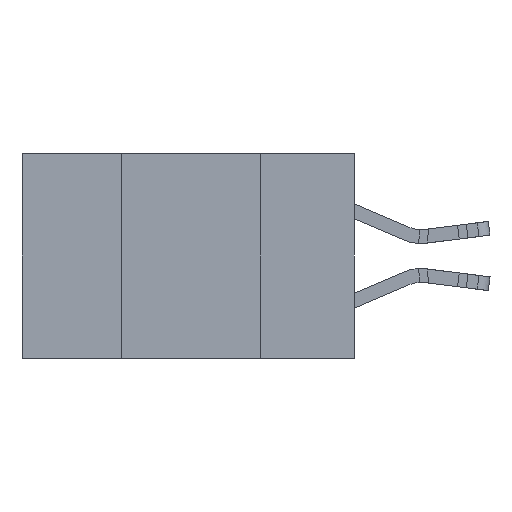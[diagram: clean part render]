
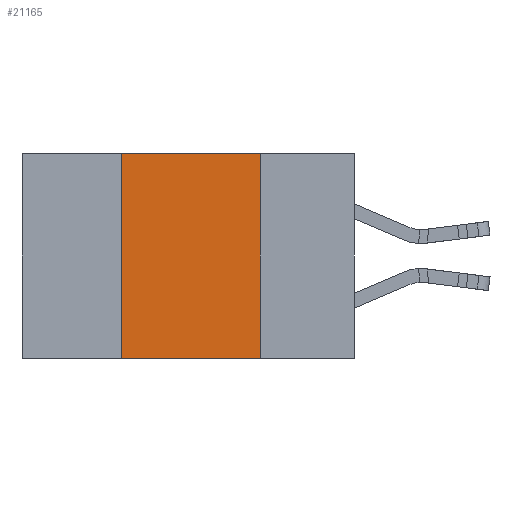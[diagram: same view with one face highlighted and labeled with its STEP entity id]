
A CAD part, left-side view. The second image highlights one B-rep face of the part: STEP entity #21165.
In plain terms, the highlighted planar face has unit normal (-1, 0, 0).
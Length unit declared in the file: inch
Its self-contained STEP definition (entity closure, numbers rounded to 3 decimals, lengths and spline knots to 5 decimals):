
#980 = ORIENTED_EDGE ( 'NONE', *, *, #19626, .T. ) ;
#2289 = ORIENTED_EDGE ( 'NONE', *, *, #3770, .F. ) ;
#3202 = VECTOR ( 'NONE', #24590, 39.37008 ) ;
#3365 = AXIS2_PLACEMENT_3D ( 'NONE', #32123, #9654, #14786 ) ;
#3557 = ORIENTED_EDGE ( 'NONE', *, *, #28721, .F. ) ;
#3770 = EDGE_CURVE ( 'NONE', #24191, #9089, #25655, .T. ) ;
#5657 = CARTESIAN_POINT ( 'NONE',  ( 0., 0.6, 0. ) ) ;
#6574 = CARTESIAN_POINT ( 'NONE',  ( 0., 0.42, -0.37 ) ) ;
#7060 = CARTESIAN_POINT ( 'NONE',  ( 0., 0.42, 0. ) ) ;
#9089 = VERTEX_POINT ( 'NONE', #14503 ) ;
#9654 = DIRECTION ( 'NONE',  ( 1., 0., 0. ) ) ;
#10833 = CARTESIAN_POINT ( 'NONE',  ( 0., 0.17, -0.37 ) ) ;
#10866 = CARTESIAN_POINT ( 'NONE',  ( 0., 0.42, 0. ) ) ;
#11649 = DIRECTION ( 'NONE',  ( 0., -1., 0. ) ) ;
#11809 = EDGE_LOOP ( 'NONE', ( #31295, #2289, #3557, #980 ) ) ;
#12265 = PLANE ( 'NONE',  #3365 ) ;
#14009 = FACE_OUTER_BOUND ( 'NONE', #11809, .T. ) ;
#14503 = CARTESIAN_POINT ( 'NONE',  ( 0., 0.17, 0. ) ) ;
#14786 = DIRECTION ( 'NONE',  ( 0., 0., -1. ) ) ;
#14924 = LINE ( 'NONE', #7060, #3202 ) ;
#15741 = DIRECTION ( 'NONE',  ( 0., -1., 0. ) ) ;
#16377 = CARTESIAN_POINT ( 'NONE',  ( 0., 0.6, -0.37 ) ) ;
#16474 = VERTEX_POINT ( 'NONE', #10833 ) ;
#16563 = LINE ( 'NONE', #25776, #24457 ) ;
#17798 = EDGE_CURVE ( 'NONE', #9089, #16474, #16563, .T. ) ;
#18997 = VECTOR ( 'NONE', #15741, 39.37008 ) ;
#19626 = EDGE_CURVE ( 'NONE', #29589, #16474, #22381, .T. ) ;
#21165 = ADVANCED_FACE ( 'NONE', ( #14009 ), #12265, .F. ) ;
#21517 = DIRECTION ( 'NONE',  ( 0., 0., -1. ) ) ;
#22352 = VECTOR ( 'NONE', #11649, 39.37008 ) ;
#22381 = LINE ( 'NONE', #16377, #22352 ) ;
#24191 = VERTEX_POINT ( 'NONE', #10866 ) ;
#24457 = VECTOR ( 'NONE', #21517, 39.37008 ) ;
#24590 = DIRECTION ( 'NONE',  ( 0., 0., 1. ) ) ;
#25655 = LINE ( 'NONE', #5657, #18997 ) ;
#25776 = CARTESIAN_POINT ( 'NONE',  ( 0., 0.17, 0. ) ) ;
#28721 = EDGE_CURVE ( 'NONE', #29589, #24191, #14924, .T. ) ;
#29589 = VERTEX_POINT ( 'NONE', #6574 ) ;
#31295 = ORIENTED_EDGE ( 'NONE', *, *, #17798, .F. ) ;
#32123 = CARTESIAN_POINT ( 'NONE',  ( 0., 0.6, 0. ) ) ;
